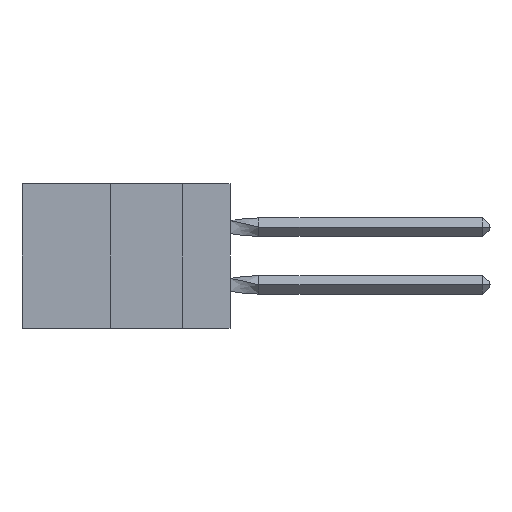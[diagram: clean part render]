
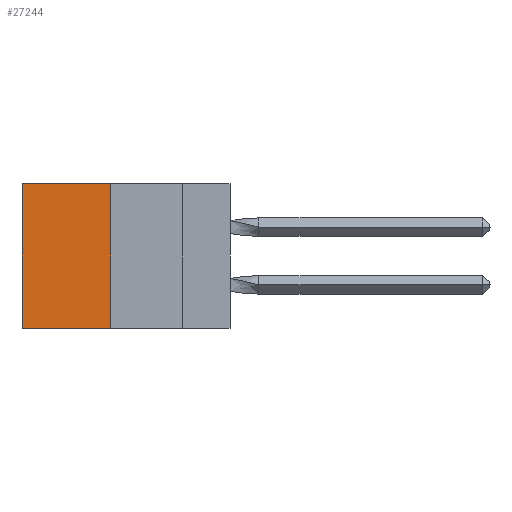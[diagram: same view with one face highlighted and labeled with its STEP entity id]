
A CAD part, left-side view. The second image highlights one B-rep face of the part: STEP entity #27244.
In plain terms, the highlighted planar face has unit normal (-1, 0, 0).
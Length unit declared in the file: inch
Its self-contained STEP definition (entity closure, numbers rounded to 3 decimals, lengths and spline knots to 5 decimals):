
#384 = VECTOR ( 'NONE', #42178, 39.37008 ) ;
#3214 = ORIENTED_EDGE ( 'NONE', *, *, #9349, .T. ) ;
#3862 = CARTESIAN_POINT ( 'NONE',  ( 0.305, 0.72, -0.5 ) ) ;
#4685 = DIRECTION ( 'NONE',  ( 1., 0., 0. ) ) ;
#4961 = CARTESIAN_POINT ( 'NONE',  ( 0.305, 0.413, -0.5 ) ) ;
#7105 = DIRECTION ( 'NONE',  ( 0., 0., -1. ) ) ;
#8084 = LINE ( 'NONE', #3862, #32998 ) ;
#8100 = CARTESIAN_POINT ( 'NONE',  ( 0.305, 0.413, -0.5 ) ) ;
#9349 = EDGE_CURVE ( 'NONE', #22555, #39429, #34629, .T. ) ;
#10879 = CARTESIAN_POINT ( 'NONE',  ( 0.305, 0.413, -0.5 ) ) ;
#10928 = AXIS2_PLACEMENT_3D ( 'NONE', #8100, #4685, #21263 ) ;
#11618 = EDGE_CURVE ( 'NONE', #39429, #21593, #8084, .T. ) ;
#13709 = VECTOR ( 'NONE', #14300, 39.37008 ) ;
#14300 = DIRECTION ( 'NONE',  ( 0., 1., 0. ) ) ;
#14711 = CARTESIAN_POINT ( 'NONE',  ( 0.305, 0.413, -0.5 ) ) ;
#16780 = CARTESIAN_POINT ( 'NONE',  ( 0.305, 0.413, 0. ) ) ;
#17027 = ORIENTED_EDGE ( 'NONE', *, *, #11618, .T. ) ;
#21122 = PLANE ( 'NONE',  #10928 ) ;
#21255 = ORIENTED_EDGE ( 'NONE', *, *, #27200, .F. ) ;
#21263 = DIRECTION ( 'NONE',  ( 0., 0., -1. ) ) ;
#21593 = VERTEX_POINT ( 'NONE', #41335 ) ;
#22080 = CARTESIAN_POINT ( 'NONE',  ( 0.305, 0.413, 0. ) ) ;
#22555 = VERTEX_POINT ( 'NONE', #22080 ) ;
#27200 = EDGE_CURVE ( 'NONE', #22555, #39704, #29092, .T. ) ;
#27244 = ADVANCED_FACE ( 'NONE', ( #30155 ), #21122, .F. ) ;
#28704 = CARTESIAN_POINT ( 'NONE',  ( 0.305, 0.72, 0. ) ) ;
#29092 = LINE ( 'NONE', #4961, #39847 ) ;
#30155 = FACE_OUTER_BOUND ( 'NONE', #36395, .T. ) ;
#31236 = DIRECTION ( 'NONE',  ( 0., 0., -1. ) ) ;
#32020 = ORIENTED_EDGE ( 'NONE', *, *, #41529, .F. ) ;
#32998 = VECTOR ( 'NONE', #7105, 39.37008 ) ;
#34629 = LINE ( 'NONE', #16780, #384 ) ;
#36395 = EDGE_LOOP ( 'NONE', ( #17027, #32020, #21255, #3214 ) ) ;
#38303 = LINE ( 'NONE', #14711, #13709 ) ;
#39429 = VERTEX_POINT ( 'NONE', #28704 ) ;
#39704 = VERTEX_POINT ( 'NONE', #10879 ) ;
#39847 = VECTOR ( 'NONE', #31236, 39.37008 ) ;
#41335 = CARTESIAN_POINT ( 'NONE',  ( 0.305, 0.72, -0.5 ) ) ;
#41529 = EDGE_CURVE ( 'NONE', #39704, #21593, #38303, .T. ) ;
#42178 = DIRECTION ( 'NONE',  ( 0., 1., 0. ) ) ;
